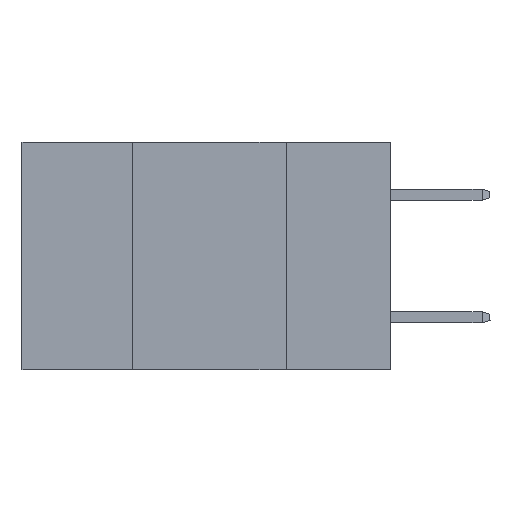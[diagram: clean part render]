
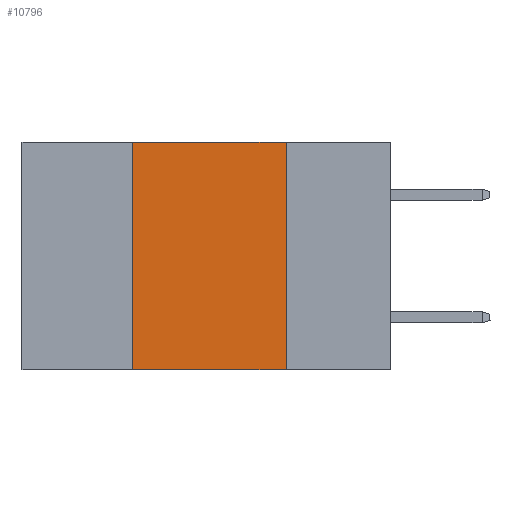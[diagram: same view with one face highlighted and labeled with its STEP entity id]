
A CAD part, left-side view. The second image highlights one B-rep face of the part: STEP entity #10796.
In plain terms, the highlighted planar face has unit normal (-1, 0, 0).
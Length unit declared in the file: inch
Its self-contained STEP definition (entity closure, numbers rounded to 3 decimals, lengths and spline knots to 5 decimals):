
#24 = DIRECTION ( 'NONE',  ( 1., 0., 0. ) ) ;
#418 = CARTESIAN_POINT ( 'NONE',  ( 0., 0.6, 0. ) ) ;
#2335 = AXIS2_PLACEMENT_3D ( 'NONE', #14586, #24, #13819 ) ;
#3194 = VERTEX_POINT ( 'NONE', #5191 ) ;
#3891 = ORIENTED_EDGE ( 'NONE', *, *, #16856, .F. ) ;
#4030 = DIRECTION ( 'NONE',  ( 0., -1., 0. ) ) ;
#4585 = CARTESIAN_POINT ( 'NONE',  ( 0., 0.6, -0.37 ) ) ;
#4657 = VERTEX_POINT ( 'NONE', #18165 ) ;
#4944 = FACE_OUTER_BOUND ( 'NONE', #4973, .T. ) ;
#4972 = VECTOR ( 'NONE', #10802, 39.37008 ) ;
#4973 = EDGE_LOOP ( 'NONE', ( #15061, #3891, #7669, #10010 ) ) ;
#5191 = CARTESIAN_POINT ( 'NONE',  ( 0., 0.17, -0.37 ) ) ;
#6312 = LINE ( 'NONE', #4585, #11766 ) ;
#7669 = ORIENTED_EDGE ( 'NONE', *, *, #8196, .F. ) ;
#8196 = EDGE_CURVE ( 'NONE', #4657, #14930, #16613, .T. ) ;
#8965 = CARTESIAN_POINT ( 'NONE',  ( 0., 0.42, 0. ) ) ;
#10010 = ORIENTED_EDGE ( 'NONE', *, *, #16859, .T. ) ;
#10289 = VERTEX_POINT ( 'NONE', #16979 ) ;
#10796 = ADVANCED_FACE ( 'NONE', ( #4944 ), #11110, .F. ) ;
#10802 = DIRECTION ( 'NONE',  ( 0., -1., 0. ) ) ;
#11110 = PLANE ( 'NONE',  #2335 ) ;
#11245 = CARTESIAN_POINT ( 'NONE',  ( 0., 0.42, 0. ) ) ;
#11766 = VECTOR ( 'NONE', #4030, 39.37008 ) ;
#12305 = VECTOR ( 'NONE', #15518, 39.37008 ) ;
#12452 = CARTESIAN_POINT ( 'NONE',  ( 0., 0.17, 0. ) ) ;
#13819 = DIRECTION ( 'NONE',  ( 0., 0., -1. ) ) ;
#14363 = VECTOR ( 'NONE', #18403, 39.37008 ) ;
#14586 = CARTESIAN_POINT ( 'NONE',  ( 0., 0.6, 0. ) ) ;
#14811 = LINE ( 'NONE', #12452, #14363 ) ;
#14930 = VERTEX_POINT ( 'NONE', #8965 ) ;
#15048 = EDGE_CURVE ( 'NONE', #10289, #3194, #14811, .T. ) ;
#15061 = ORIENTED_EDGE ( 'NONE', *, *, #15048, .F. ) ;
#15518 = DIRECTION ( 'NONE',  ( 0., 0., 1. ) ) ;
#16613 = LINE ( 'NONE', #11245, #12305 ) ;
#16793 = LINE ( 'NONE', #418, #4972 ) ;
#16856 = EDGE_CURVE ( 'NONE', #14930, #10289, #16793, .T. ) ;
#16859 = EDGE_CURVE ( 'NONE', #4657, #3194, #6312, .T. ) ;
#16979 = CARTESIAN_POINT ( 'NONE',  ( 0., 0.17, 0. ) ) ;
#18165 = CARTESIAN_POINT ( 'NONE',  ( 0., 0.42, -0.37 ) ) ;
#18403 = DIRECTION ( 'NONE',  ( 0., 0., -1. ) ) ;
